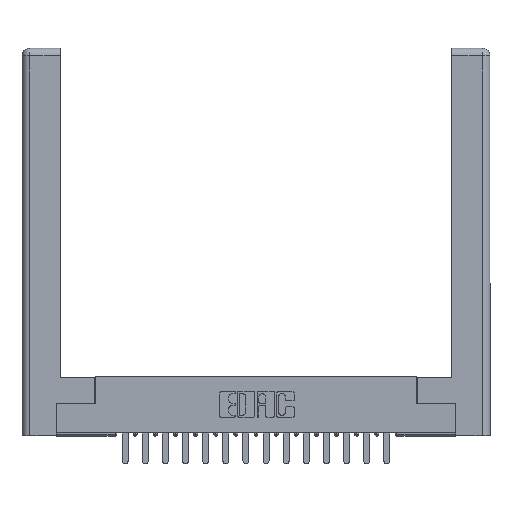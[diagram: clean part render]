
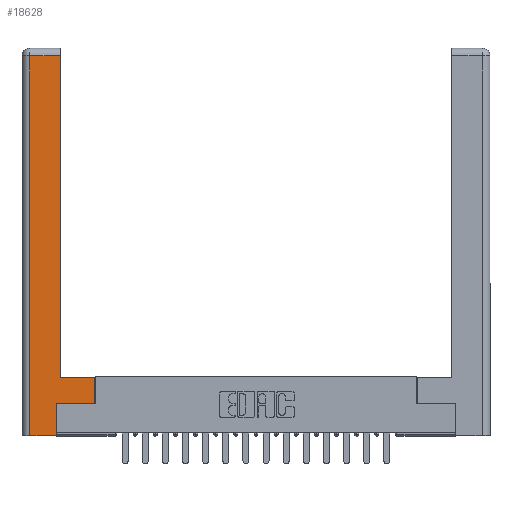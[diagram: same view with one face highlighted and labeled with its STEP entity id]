
A CAD part, top view. The second image highlights one B-rep face of the part: STEP entity #18628.
In plain terms, the highlighted planar face has unit normal (0, 0, 1).
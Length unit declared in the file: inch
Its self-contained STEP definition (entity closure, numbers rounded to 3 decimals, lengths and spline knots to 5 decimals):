
#153 = CARTESIAN_POINT ( 'NONE',  ( 0.265, 0., 0. ) ) ;
#218 = EDGE_CURVE ( 'NONE', #11943, #7021, #9971, .T. ) ;
#530 = EDGE_CURVE ( 'NONE', #5771, #3066, #12384, .T. ) ;
#1206 = DIRECTION ( 'NONE',  ( 0., 1., 0. ) ) ;
#1310 = EDGE_CURVE ( 'NONE', #6326, #5771, #1416, .T. ) ;
#1416 = LINE ( 'NONE', #153, #16493 ) ;
#2207 = VERTEX_POINT ( 'NONE', #2298 ) ;
#2298 = CARTESIAN_POINT ( 'NONE',  ( 0.295, 0.45, 0. ) ) ;
#2407 = PLANE ( 'NONE',  #14977 ) ;
#2507 = DIRECTION ( 'NONE',  ( -1., 0., 0. ) ) ;
#2614 = ORIENTED_EDGE ( 'NONE', *, *, #7568, .T. ) ;
#3066 = VERTEX_POINT ( 'NONE', #10921 ) ;
#3293 = CARTESIAN_POINT ( 'NONE',  ( 0.265, 0., 0. ) ) ;
#3537 = DIRECTION ( 'NONE',  ( 0., 1., 0. ) ) ;
#3735 = ORIENTED_EDGE ( 'NONE', *, *, #17915, .T. ) ;
#3850 = CARTESIAN_POINT ( 'NONE',  ( 0.295, 0.45, 0. ) ) ;
#4844 = ORIENTED_EDGE ( 'NONE', *, *, #1310, .T. ) ;
#5399 = LINE ( 'NONE', #14541, #6206 ) ;
#5425 = CARTESIAN_POINT ( 'NONE',  ( 0., 0., 0. ) ) ;
#5771 = VERTEX_POINT ( 'NONE', #3293 ) ;
#5952 = EDGE_CURVE ( 'NONE', #7021, #2207, #17215, .T. ) ;
#5955 = ORIENTED_EDGE ( 'NONE', *, *, #14320, .T. ) ;
#6206 = VECTOR ( 'NONE', #13277, 39.37008 ) ;
#6326 = VERTEX_POINT ( 'NONE', #14236 ) ;
#6545 = CARTESIAN_POINT ( 'NONE',  ( 0.265, 0.245, 0. ) ) ;
#6680 = VECTOR ( 'NONE', #9791, 39.37008 ) ;
#6746 = CARTESIAN_POINT ( 'NONE',  ( 0.295, 2.94, 0. ) ) ;
#6986 = FACE_OUTER_BOUND ( 'NONE', #19026, .T. ) ;
#7021 = VERTEX_POINT ( 'NONE', #17949 ) ;
#7511 = LINE ( 'NONE', #10026, #15634 ) ;
#7568 = EDGE_CURVE ( 'NONE', #2207, #11334, #11515, .T. ) ;
#8226 = EDGE_CURVE ( 'NONE', #3066, #11943, #7511, .T. ) ;
#8392 = ORIENTED_EDGE ( 'NONE', *, *, #218, .T. ) ;
#8649 = VECTOR ( 'NONE', #3537, 39.37008 ) ;
#9791 = DIRECTION ( 'NONE',  ( -1., 0., 0. ) ) ;
#9853 = VECTOR ( 'NONE', #13217, 39.37008 ) ;
#9971 = LINE ( 'NONE', #11527, #16767 ) ;
#10026 = CARTESIAN_POINT ( 'NONE',  ( 0.565, 0.245, 0. ) ) ;
#10921 = CARTESIAN_POINT ( 'NONE',  ( 0.265, 0.245, 0. ) ) ;
#11334 = VERTEX_POINT ( 'NONE', #6746 ) ;
#11515 = LINE ( 'NONE', #14050, #15300 ) ;
#11527 = CARTESIAN_POINT ( 'NONE',  ( 0.565, 0.45, 0. ) ) ;
#11943 = VERTEX_POINT ( 'NONE', #17820 ) ;
#12384 = LINE ( 'NONE', #6545, #8649 ) ;
#12683 = DIRECTION ( 'NONE',  ( 0., 1., 0. ) ) ;
#13119 = LINE ( 'NONE', #17533, #9853 ) ;
#13217 = DIRECTION ( 'NONE',  ( 0., -1., 0. ) ) ;
#13277 = DIRECTION ( 'NONE',  ( -1., 0., 0. ) ) ;
#13334 = DIRECTION ( 'NONE',  ( 1., 0., 0. ) ) ;
#13610 = CARTESIAN_POINT ( 'NONE',  ( 0.0615, 2.94, 0. ) ) ;
#14050 = CARTESIAN_POINT ( 'NONE',  ( 0.295, 3., 0. ) ) ;
#14236 = CARTESIAN_POINT ( 'NONE',  ( 0.0615, 0., 0. ) ) ;
#14247 = ORIENTED_EDGE ( 'NONE', *, *, #5952, .T. ) ;
#14320 = EDGE_CURVE ( 'NONE', #15753, #6326, #13119, .T. ) ;
#14541 = CARTESIAN_POINT ( 'NONE',  ( 0.0615, 2.94, 0. ) ) ;
#14977 = AXIS2_PLACEMENT_3D ( 'NONE', #5425, #17233, #2507 ) ;
#15036 = DIRECTION ( 'NONE',  ( 1., 0., 0. ) ) ;
#15300 = VECTOR ( 'NONE', #12683, 39.37008 ) ;
#15634 = VECTOR ( 'NONE', #13334, 39.37008 ) ;
#15753 = VERTEX_POINT ( 'NONE', #13610 ) ;
#16308 = ORIENTED_EDGE ( 'NONE', *, *, #530, .T. ) ;
#16493 = VECTOR ( 'NONE', #15036, 39.37008 ) ;
#16767 = VECTOR ( 'NONE', #1206, 39.37008 ) ;
#17215 = LINE ( 'NONE', #3850, #6680 ) ;
#17233 = DIRECTION ( 'NONE',  ( 0., 0., -1. ) ) ;
#17533 = CARTESIAN_POINT ( 'NONE',  ( 0.0615, 0., 0. ) ) ;
#17820 = CARTESIAN_POINT ( 'NONE',  ( 0.565, 0.245, 0. ) ) ;
#17915 = EDGE_CURVE ( 'NONE', #11334, #15753, #5399, .T. ) ;
#17949 = CARTESIAN_POINT ( 'NONE',  ( 0.565, 0.45, 0. ) ) ;
#18628 = ADVANCED_FACE ( 'NONE', ( #6986 ), #2407, .F. ) ;
#18831 = ORIENTED_EDGE ( 'NONE', *, *, #8226, .T. ) ;
#19026 = EDGE_LOOP ( 'NONE', ( #2614, #3735, #5955, #4844, #16308, #18831, #8392, #14247 ) ) ;
